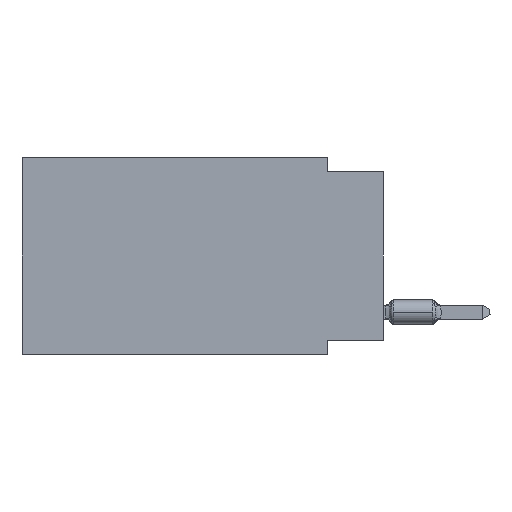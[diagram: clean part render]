
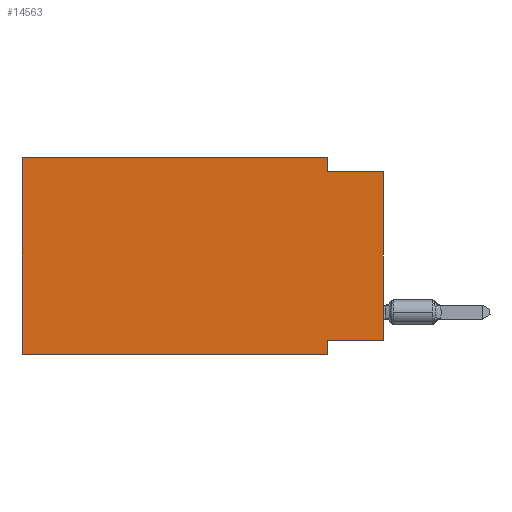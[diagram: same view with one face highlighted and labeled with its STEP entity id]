
A CAD part, left-side view. The second image highlights one B-rep face of the part: STEP entity #14563.
In plain terms, the highlighted planar face has unit normal (-1, 0, 0).
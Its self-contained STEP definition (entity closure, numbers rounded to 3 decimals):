
#1088 = CARTESIAN_POINT ( 'NONE',  ( 0., 0., -8.255 ) ) ;
#1181 = EDGE_LOOP ( 'NONE', ( #27009, #20919, #12044, #36305, #9350, #12397, #28473, #21469 ) ) ;
#2477 = LINE ( 'NONE', #28775, #11620 ) ;
#3098 = VECTOR ( 'NONE', #3329, 1000. ) ;
#3329 = DIRECTION ( 'NONE',  ( 0., 0., -1. ) ) ;
#4297 = VERTEX_POINT ( 'NONE', #26474 ) ;
#4935 = DIRECTION ( 'NONE',  ( 0., 0., -1. ) ) ;
#4966 = VERTEX_POINT ( 'NONE', #16097 ) ;
#5072 = VECTOR ( 'NONE', #38896, 1000. ) ;
#6795 = VERTEX_POINT ( 'NONE', #35689 ) ;
#7806 = DIRECTION ( 'NONE',  ( 0., 0., 1. ) ) ;
#8737 = EDGE_CURVE ( 'NONE', #4297, #30780, #22097, .T. ) ;
#9256 = CARTESIAN_POINT ( 'NONE',  ( 0., 16.383, -8.89 ) ) ;
#9350 = ORIENTED_EDGE ( 'NONE', *, *, #22123, .F. ) ;
#9388 = LINE ( 'NONE', #1088, #27893 ) ;
#9879 = DIRECTION ( 'NONE',  ( 0., 0., -1. ) ) ;
#10385 = DIRECTION ( 'NONE',  ( 0., 0., 1. ) ) ;
#11073 = PLANE ( 'NONE',  #18332 ) ;
#11620 = VECTOR ( 'NONE', #26584, 1000. ) ;
#11728 = DIRECTION ( 'NONE',  ( 0., -1., 0. ) ) ;
#12044 = ORIENTED_EDGE ( 'NONE', *, *, #8737, .F. ) ;
#12098 = EDGE_CURVE ( 'NONE', #30780, #20318, #23888, .T. ) ;
#12397 = ORIENTED_EDGE ( 'NONE', *, *, #36341, .T. ) ;
#14563 = ADVANCED_FACE ( 'NONE', ( #29843 ), #11073, .F. ) ;
#15226 = CARTESIAN_POINT ( 'NONE',  ( 0., 16.383, 0. ) ) ;
#15329 = DIRECTION ( 'NONE',  ( 0., 1., 0. ) ) ;
#16097 = CARTESIAN_POINT ( 'NONE',  ( 0., 0., -8.255 ) ) ;
#17343 = VECTOR ( 'NONE', #11728, 1000. ) ;
#17477 = LINE ( 'NONE', #35248, #21695 ) ;
#18332 = AXIS2_PLACEMENT_3D ( 'NONE', #23137, #26468, #4935 ) ;
#18542 = CARTESIAN_POINT ( 'NONE',  ( 0., 0., -0.635 ) ) ;
#18766 = CARTESIAN_POINT ( 'NONE',  ( 0., 2.54, -8.89 ) ) ;
#19082 = VECTOR ( 'NONE', #10385, 1000. ) ;
#20318 = VERTEX_POINT ( 'NONE', #30653 ) ;
#20919 = ORIENTED_EDGE ( 'NONE', *, *, #12098, .F. ) ;
#21303 = VERTEX_POINT ( 'NONE', #28656 ) ;
#21469 = ORIENTED_EDGE ( 'NONE', *, *, #21966, .F. ) ;
#21695 = VECTOR ( 'NONE', #7806, 1000. ) ;
#21966 = EDGE_CURVE ( 'NONE', #4966, #6795, #9388, .T. ) ;
#22097 = LINE ( 'NONE', #27230, #3098 ) ;
#22123 = EDGE_CURVE ( 'NONE', #38283, #22269, #31502, .T. ) ;
#22269 = VERTEX_POINT ( 'NONE', #15226 ) ;
#22303 = VECTOR ( 'NONE', #9879, 1000. ) ;
#22626 = CARTESIAN_POINT ( 'NONE',  ( 0., 16.383, 0. ) ) ;
#23137 = CARTESIAN_POINT ( 'NONE',  ( 0., 16.383, 0. ) ) ;
#23888 = LINE ( 'NONE', #18542, #5072 ) ;
#26468 = DIRECTION ( 'NONE',  ( 1., 0., 0. ) ) ;
#26474 = CARTESIAN_POINT ( 'NONE',  ( 0., 2.54, 0. ) ) ;
#26584 = DIRECTION ( 'NONE',  ( 0., -1., 0. ) ) ;
#26749 = CARTESIAN_POINT ( 'NONE',  ( 0., 16.383, 0. ) ) ;
#27009 = ORIENTED_EDGE ( 'NONE', *, *, #29495, .T. ) ;
#27230 = CARTESIAN_POINT ( 'NONE',  ( 0., 2.54, 0. ) ) ;
#27893 = VECTOR ( 'NONE', #15329, 1000. ) ;
#28473 = ORIENTED_EDGE ( 'NONE', *, *, #33192, .F. ) ;
#28656 = CARTESIAN_POINT ( 'NONE',  ( 0., 2.54, -8.89 ) ) ;
#28775 = CARTESIAN_POINT ( 'NONE',  ( 0., 16.383, -8.89 ) ) ;
#29495 = EDGE_CURVE ( 'NONE', #4966, #20318, #17477, .T. ) ;
#29843 = FACE_OUTER_BOUND ( 'NONE', #1181, .T. ) ;
#30653 = CARTESIAN_POINT ( 'NONE',  ( 0., 0., -0.635 ) ) ;
#30780 = VERTEX_POINT ( 'NONE', #39033 ) ;
#31502 = LINE ( 'NONE', #22626, #19082 ) ;
#33192 = EDGE_CURVE ( 'NONE', #6795, #21303, #34389, .T. ) ;
#33243 = LINE ( 'NONE', #26749, #17343 ) ;
#34389 = LINE ( 'NONE', #18766, #22303 ) ;
#35248 = CARTESIAN_POINT ( 'NONE',  ( 0., 0., 0. ) ) ;
#35689 = CARTESIAN_POINT ( 'NONE',  ( 0., 2.54, -8.255 ) ) ;
#36305 = ORIENTED_EDGE ( 'NONE', *, *, #36839, .F. ) ;
#36341 = EDGE_CURVE ( 'NONE', #38283, #21303, #2477, .T. ) ;
#36839 = EDGE_CURVE ( 'NONE', #22269, #4297, #33243, .T. ) ;
#38283 = VERTEX_POINT ( 'NONE', #9256 ) ;
#38896 = DIRECTION ( 'NONE',  ( 0., -1., 0. ) ) ;
#39033 = CARTESIAN_POINT ( 'NONE',  ( 0., 2.54, -0.635 ) ) ;
